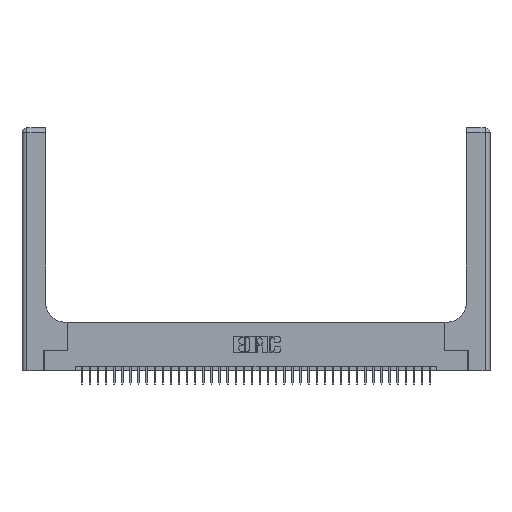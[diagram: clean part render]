
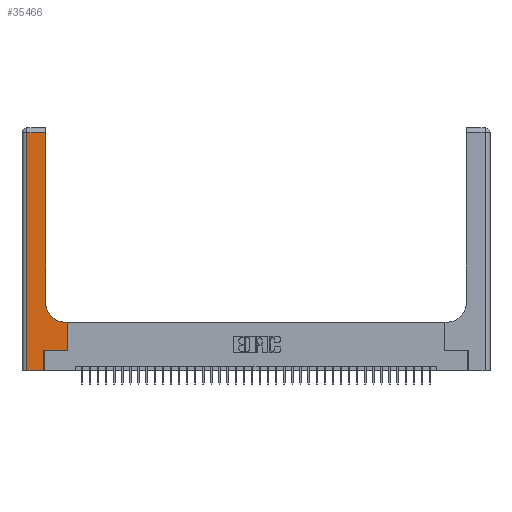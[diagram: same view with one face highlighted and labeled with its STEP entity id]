
A CAD part, top view. The second image highlights one B-rep face of the part: STEP entity #35466.
In plain terms, the highlighted planar face has unit normal (0, 0, 1).
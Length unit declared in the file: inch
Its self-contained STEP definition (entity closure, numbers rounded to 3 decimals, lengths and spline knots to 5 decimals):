
#370 = VECTOR ( 'NONE', #39258, 39.37008 ) ;
#558 = DIRECTION ( 'NONE',  ( -1., 0., 0. ) ) ;
#1712 = EDGE_LOOP ( 'NONE', ( #11666, #19261, #20003, #33051, #9281, #28433, #10086, #34511, #37136 ) ) ;
#2893 = VECTOR ( 'NONE', #3106, 39.37008 ) ;
#3106 = DIRECTION ( 'NONE',  ( 0., 1., 0. ) ) ;
#3361 = EDGE_CURVE ( 'NONE', #13495, #28336, #15155, .T. ) ;
#3588 = CARTESIAN_POINT ( 'NONE',  ( 0.5585, 0.25, 0.37 ) ) ;
#5158 = EDGE_CURVE ( 'NONE', #18509, #14181, #21946, .T. ) ;
#5588 = VECTOR ( 'NONE', #21217, 39.37008 ) ;
#6018 = LINE ( 'NONE', #38372, #22669 ) ;
#6483 = DIRECTION ( 'NONE',  ( 0., 0., -1. ) ) ;
#6879 = PLANE ( 'NONE',  #34172 ) ;
#7950 = LINE ( 'NONE', #33363, #5588 ) ;
#8220 = CARTESIAN_POINT ( 'NONE',  ( 0.06, 0., 0.37 ) ) ;
#8429 = DIRECTION ( 'NONE',  ( 1., 0., 0. ) ) ;
#9281 = ORIENTED_EDGE ( 'NONE', *, *, #22501, .T. ) ;
#9347 = EDGE_CURVE ( 'NONE', #34924, #18509, #20193, .T. ) ;
#9425 = VECTOR ( 'NONE', #8429, 39.37008 ) ;
#10086 = ORIENTED_EDGE ( 'NONE', *, *, #3361, .T. ) ;
#11009 = CARTESIAN_POINT ( 'NONE',  ( 0.5415, 0.85, 0.37 ) ) ;
#11666 = ORIENTED_EDGE ( 'NONE', *, *, #5158, .T. ) ;
#12304 = DIRECTION ( 'NONE',  ( 0., 1., 0. ) ) ;
#12327 = CARTESIAN_POINT ( 'NONE',  ( 0.2915, 3., 0.37 ) ) ;
#12670 = CARTESIAN_POINT ( 'NONE',  ( 0., 0., 0.37 ) ) ;
#13117 = VERTEX_POINT ( 'NONE', #16464 ) ;
#13228 = EDGE_CURVE ( 'NONE', #15047, #13117, #37427, .T. ) ;
#13495 = VERTEX_POINT ( 'NONE', #31453 ) ;
#13963 = DIRECTION ( 'NONE',  ( 1., 0., 0. ) ) ;
#14181 = VERTEX_POINT ( 'NONE', #30273 ) ;
#14732 = CARTESIAN_POINT ( 'NONE',  ( 0., 2.94, 0.37 ) ) ;
#15047 = VERTEX_POINT ( 'NONE', #8220 ) ;
#15155 = LINE ( 'NONE', #3588, #39481 ) ;
#15381 = DIRECTION ( 'NONE',  ( 1., 0., 0. ) ) ;
#15708 = LINE ( 'NONE', #14732, #370 ) ;
#16386 = AXIS2_PLACEMENT_3D ( 'NONE', #11009, #35848, #13963 ) ;
#16464 = CARTESIAN_POINT ( 'NONE',  ( 0.269, 0., 0.37 ) ) ;
#16600 = LINE ( 'NONE', #39229, #9425 ) ;
#17324 = CARTESIAN_POINT ( 'NONE',  ( 0.06, 2.94, 0.37 ) ) ;
#17935 = VECTOR ( 'NONE', #15381, 39.37008 ) ;
#18434 = DIRECTION ( 'NONE',  ( 0., 1., 0. ) ) ;
#18509 = VERTEX_POINT ( 'NONE', #32661 ) ;
#19261 = ORIENTED_EDGE ( 'NONE', *, *, #39302, .T. ) ;
#19469 = CARTESIAN_POINT ( 'NONE',  ( 0.5585, 0.6, 0.37 ) ) ;
#20003 = ORIENTED_EDGE ( 'NONE', *, *, #33725, .T. ) ;
#20193 = CIRCLE ( 'NONE', #16386, 0.25 ) ;
#21179 = EDGE_CURVE ( 'NONE', #35962, #13495, #16600, .T. ) ;
#21217 = DIRECTION ( 'NONE',  ( -1., 0., 0. ) ) ;
#21946 = LINE ( 'NONE', #12327, #2893 ) ;
#22501 = EDGE_CURVE ( 'NONE', #13117, #35962, #31751, .T. ) ;
#22669 = VECTOR ( 'NONE', #28885, 39.37008 ) ;
#22943 = CARTESIAN_POINT ( 'NONE',  ( 0.269, 0.25, 0.37 ) ) ;
#28336 = VERTEX_POINT ( 'NONE', #19469 ) ;
#28433 = ORIENTED_EDGE ( 'NONE', *, *, #21179, .T. ) ;
#28885 = DIRECTION ( 'NONE',  ( 0., -1., 0. ) ) ;
#29394 = VECTOR ( 'NONE', #12304, 39.37008 ) ;
#29513 = VERTEX_POINT ( 'NONE', #17324 ) ;
#30273 = CARTESIAN_POINT ( 'NONE',  ( 0.2915, 2.94, 0.37 ) ) ;
#30516 = CARTESIAN_POINT ( 'NONE',  ( 0.269, 0., 0.37 ) ) ;
#31453 = CARTESIAN_POINT ( 'NONE',  ( 0.5585, 0.25, 0.37 ) ) ;
#31751 = LINE ( 'NONE', #30516, #29394 ) ;
#32661 = CARTESIAN_POINT ( 'NONE',  ( 0.2915, 0.85, 0.37 ) ) ;
#33051 = ORIENTED_EDGE ( 'NONE', *, *, #13228, .T. ) ;
#33363 = CARTESIAN_POINT ( 'NONE',  ( 0.2915, 0.6, 0.37 ) ) ;
#33402 = EDGE_CURVE ( 'NONE', #28336, #34924, #7950, .T. ) ;
#33725 = EDGE_CURVE ( 'NONE', #29513, #15047, #6018, .T. ) ;
#34172 = AXIS2_PLACEMENT_3D ( 'NONE', #37014, #6483, #558 ) ;
#34316 = CARTESIAN_POINT ( 'NONE',  ( 0.5415, 0.6, 0.37 ) ) ;
#34511 = ORIENTED_EDGE ( 'NONE', *, *, #33402, .T. ) ;
#34924 = VERTEX_POINT ( 'NONE', #34316 ) ;
#35466 = ADVANCED_FACE ( 'NONE', ( #36008 ), #6879, .F. ) ;
#35848 = DIRECTION ( 'NONE',  ( 0., 0., -1. ) ) ;
#35962 = VERTEX_POINT ( 'NONE', #22943 ) ;
#36008 = FACE_OUTER_BOUND ( 'NONE', #1712, .T. ) ;
#37014 = CARTESIAN_POINT ( 'NONE',  ( 0., 3., 0.37 ) ) ;
#37136 = ORIENTED_EDGE ( 'NONE', *, *, #9347, .T. ) ;
#37427 = LINE ( 'NONE', #12670, #17935 ) ;
#38372 = CARTESIAN_POINT ( 'NONE',  ( 0.06, 3., 0.37 ) ) ;
#39229 = CARTESIAN_POINT ( 'NONE',  ( 0.269, 0.25, 0.37 ) ) ;
#39258 = DIRECTION ( 'NONE',  ( -1., 0., 0. ) ) ;
#39302 = EDGE_CURVE ( 'NONE', #14181, #29513, #15708, .T. ) ;
#39481 = VECTOR ( 'NONE', #18434, 39.37008 ) ;
